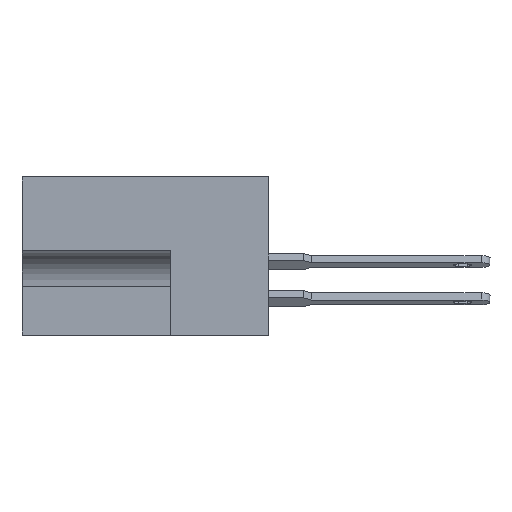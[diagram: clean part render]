
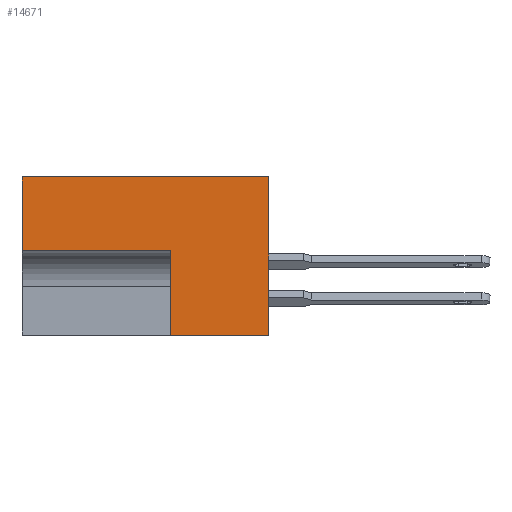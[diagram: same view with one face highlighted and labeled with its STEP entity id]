
A CAD part, left-side view. The second image highlights one B-rep face of the part: STEP entity #14671.
In plain terms, the highlighted planar face has unit normal (-1, 0, 0).
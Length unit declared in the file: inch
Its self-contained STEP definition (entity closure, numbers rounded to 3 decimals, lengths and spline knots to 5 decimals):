
#57 = ORIENTED_EDGE ( 'NONE', *, *, #11447, .T. ) ;
#133 = LINE ( 'NONE', #13720, #2866 ) ;
#588 = VERTEX_POINT ( 'NONE', #10405 ) ;
#745 = VERTEX_POINT ( 'NONE', #14829 ) ;
#996 = CARTESIAN_POINT ( 'NONE',  ( 0., 0., 0. ) ) ;
#1417 = EDGE_CURVE ( 'NONE', #745, #588, #133, .T. ) ;
#1478 = DIRECTION ( 'NONE',  ( 0., 1., 0. ) ) ;
#1987 = EDGE_CURVE ( 'NONE', #8395, #10774, #2848, .T. ) ;
#2054 = CARTESIAN_POINT ( 'NONE',  ( 0., 0., 0. ) ) ;
#2230 = EDGE_CURVE ( 'NONE', #588, #15659, #9132, .T. ) ;
#2848 = LINE ( 'NONE', #2054, #15808 ) ;
#2866 = VECTOR ( 'NONE', #3446, 39.37008 ) ;
#3198 = ORIENTED_EDGE ( 'NONE', *, *, #12405, .F. ) ;
#3204 = AXIS2_PLACEMENT_3D ( 'NONE', #6532, #12772, #13929 ) ;
#3446 = DIRECTION ( 'NONE',  ( 0., 0., 1. ) ) ;
#3800 = LINE ( 'NONE', #13362, #15580 ) ;
#3860 = EDGE_CURVE ( 'NONE', #12414, #10774, #10879, .T. ) ;
#4568 = CARTESIAN_POINT ( 'NONE',  ( 0., 0.828, -0.248 ) ) ;
#4799 = DIRECTION ( 'NONE',  ( 0., 0., 1. ) ) ;
#6283 = DIRECTION ( 'NONE',  ( 0., -1., 0. ) ) ;
#6532 = CARTESIAN_POINT ( 'NONE',  ( 0., 0.453, 0. ) ) ;
#6906 = ORIENTED_EDGE ( 'NONE', *, *, #1987, .T. ) ;
#7810 = ORIENTED_EDGE ( 'NONE', *, *, #1417, .F. ) ;
#8395 = VERTEX_POINT ( 'NONE', #14982 ) ;
#9132 = LINE ( 'NONE', #10138, #12485 ) ;
#9613 = DIRECTION ( 'NONE',  ( 0., 0., 1. ) ) ;
#10138 = CARTESIAN_POINT ( 'NONE',  ( 0., 0.328, -0.248 ) ) ;
#10258 = PLANE ( 'NONE',  #3204 ) ;
#10405 = CARTESIAN_POINT ( 'NONE',  ( 0., 0.328, -0.248 ) ) ;
#10472 = ORIENTED_EDGE ( 'NONE', *, *, #2230, .F. ) ;
#10774 = VERTEX_POINT ( 'NONE', #996 ) ;
#10879 = LINE ( 'NONE', #13836, #13434 ) ;
#11311 = ORIENTED_EDGE ( 'NONE', *, *, #3860, .F. ) ;
#11447 = EDGE_CURVE ( 'NONE', #745, #8395, #15414, .T. ) ;
#12266 = CARTESIAN_POINT ( 'NONE',  ( 0., 0.828, 0. ) ) ;
#12405 = EDGE_CURVE ( 'NONE', #15659, #12414, #3800, .T. ) ;
#12414 = VERTEX_POINT ( 'NONE', #12266 ) ;
#12485 = VECTOR ( 'NONE', #1478, 39.37008 ) ;
#12772 = DIRECTION ( 'NONE',  ( 1., 0., 0. ) ) ;
#12943 = DIRECTION ( 'NONE',  ( 0., -1., 0. ) ) ;
#13004 = CARTESIAN_POINT ( 'NONE',  ( 0., 0.453, -0.531 ) ) ;
#13290 = VECTOR ( 'NONE', #12943, 39.37008 ) ;
#13362 = CARTESIAN_POINT ( 'NONE',  ( 0., 0.828, 0. ) ) ;
#13434 = VECTOR ( 'NONE', #6283, 39.37008 ) ;
#13673 = FACE_OUTER_BOUND ( 'NONE', #14460, .T. ) ;
#13720 = CARTESIAN_POINT ( 'NONE',  ( 0., 0.328, -0.531 ) ) ;
#13836 = CARTESIAN_POINT ( 'NONE',  ( 0., 0.453, 0. ) ) ;
#13929 = DIRECTION ( 'NONE',  ( 0., 0., -1. ) ) ;
#14460 = EDGE_LOOP ( 'NONE', ( #3198, #10472, #7810, #57, #6906, #11311 ) ) ;
#14671 = ADVANCED_FACE ( 'NONE', ( #13673 ), #10258, .F. ) ;
#14829 = CARTESIAN_POINT ( 'NONE',  ( 0., 0.328, -0.531 ) ) ;
#14982 = CARTESIAN_POINT ( 'NONE',  ( 0., 0., -0.531 ) ) ;
#15414 = LINE ( 'NONE', #13004, #13290 ) ;
#15580 = VECTOR ( 'NONE', #4799, 39.37008 ) ;
#15659 = VERTEX_POINT ( 'NONE', #4568 ) ;
#15808 = VECTOR ( 'NONE', #9613, 39.37008 ) ;
